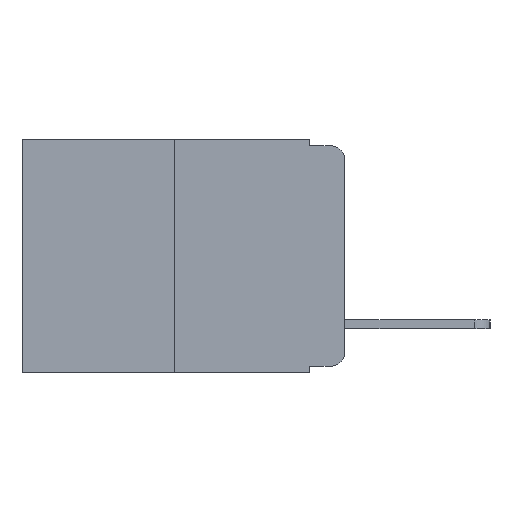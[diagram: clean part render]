
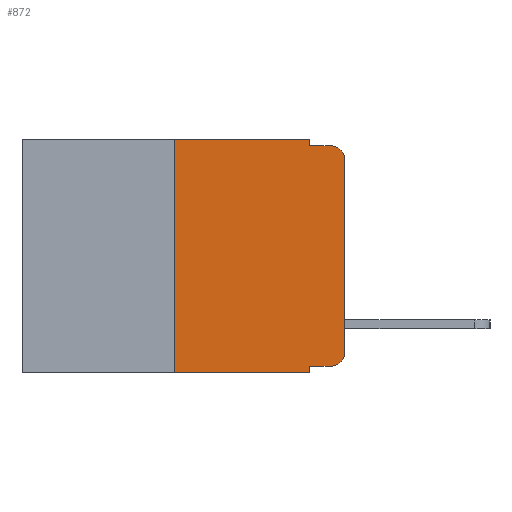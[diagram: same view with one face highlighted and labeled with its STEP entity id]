
A CAD part, left-side view. The second image highlights one B-rep face of the part: STEP entity #872.
In plain terms, the highlighted planar face has unit normal (-1, 0, 0).
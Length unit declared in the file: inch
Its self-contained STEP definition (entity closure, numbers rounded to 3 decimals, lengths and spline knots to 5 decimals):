
#131 = DIRECTION ( 'NONE',  ( 0., 0., -1. ) ) ;
#144 = EDGE_CURVE ( 'NONE', #8799, #7692, #14751, .T. ) ;
#221 = EDGE_LOOP ( 'NONE', ( #7815, #8333, #8622, #9562, #9704, #9836, #9785, #9309, #9465, #8725 ) ) ;
#251 = EDGE_CURVE ( 'NONE', #6473, #8799, #6221, .T. ) ;
#286 = CARTESIAN_POINT ( 'NONE',  ( 0., 0.051, 0. ) ) ;
#451 = VECTOR ( 'NONE', #1608, 39.37008 ) ;
#872 = ADVANCED_FACE ( 'NONE', ( #10704 ), #4887, .F. ) ;
#1161 = EDGE_CURVE ( 'NONE', #7692, #6128, #2024, .T. ) ;
#1162 = CARTESIAN_POINT ( 'NONE',  ( 0., 0.051, -0.343 ) ) ;
#1356 = CARTESIAN_POINT ( 'NONE',  ( 0., 0.25, 0. ) ) ;
#1543 = VERTEX_POINT ( 'NONE', #7859 ) ;
#1608 = DIRECTION ( 'NONE',  ( 0., 0., -1. ) ) ;
#1846 = CARTESIAN_POINT ( 'NONE',  ( 0., 0.02, -0.313 ) ) ;
#1879 = DIRECTION ( 'NONE',  ( 0., 0., 1. ) ) ;
#1979 = EDGE_CURVE ( 'NONE', #6128, #7221, #2002, .T. ) ;
#2002 = LINE ( 'NONE', #9554, #7936 ) ;
#2024 = LINE ( 'NONE', #8355, #13889 ) ;
#2084 = CARTESIAN_POINT ( 'NONE',  ( 0., 0.051, -0.333 ) ) ;
#2280 = CARTESIAN_POINT ( 'NONE',  ( 0., 0.473, 0. ) ) ;
#2773 = EDGE_CURVE ( 'NONE', #11988, #7221, #12708, .T. ) ;
#3029 = DIRECTION ( 'NONE',  ( 0., 0., -1. ) ) ;
#3569 = EDGE_CURVE ( 'NONE', #5573, #11988, #11482, .T. ) ;
#3654 = AXIS2_PLACEMENT_3D ( 'NONE', #1846, #10107, #3029 ) ;
#4259 = CARTESIAN_POINT ( 'NONE',  ( 0., 0., -0.313 ) ) ;
#4367 = DIRECTION ( 'NONE',  ( 0., -1., 0. ) ) ;
#4872 = EDGE_CURVE ( 'NONE', #6473, #12690, #12657, .T. ) ;
#4887 = PLANE ( 'NONE',  #13599 ) ;
#5160 = VERTEX_POINT ( 'NONE', #2084 ) ;
#5573 = VERTEX_POINT ( 'NONE', #4259 ) ;
#5961 = CARTESIAN_POINT ( 'NONE',  ( 0., 0., -0.03 ) ) ;
#6128 = VERTEX_POINT ( 'NONE', #11013 ) ;
#6221 = LINE ( 'NONE', #1356, #8914 ) ;
#6473 = VERTEX_POINT ( 'NONE', #9425 ) ;
#6611 = VECTOR ( 'NONE', #8003, 39.37008 ) ;
#6870 = CARTESIAN_POINT ( 'NONE',  ( 0., 0.473, -0.343 ) ) ;
#7221 = VERTEX_POINT ( 'NONE', #7530 ) ;
#7399 = DIRECTION ( 'NONE',  ( -1., 0., 0. ) ) ;
#7530 = CARTESIAN_POINT ( 'NONE',  ( 0., 0.02, -0.01 ) ) ;
#7692 = VERTEX_POINT ( 'NONE', #12306 ) ;
#7787 = CARTESIAN_POINT ( 'NONE',  ( 0., 0., 0. ) ) ;
#7815 = ORIENTED_EDGE ( 'NONE', *, *, #3569, .T. ) ;
#7859 = CARTESIAN_POINT ( 'NONE',  ( 0., 0.02, -0.333 ) ) ;
#7889 = CARTESIAN_POINT ( 'NONE',  ( 0., 0.051, -0.333 ) ) ;
#7936 = VECTOR ( 'NONE', #14992, 39.37008 ) ;
#8003 = DIRECTION ( 'NONE',  ( 0., -1., 0. ) ) ;
#8333 = ORIENTED_EDGE ( 'NONE', *, *, #2773, .T. ) ;
#8336 = DIRECTION ( 'NONE',  ( 0., 0., -1. ) ) ;
#8355 = CARTESIAN_POINT ( 'NONE',  ( 0., 0.051, 0. ) ) ;
#8438 = VECTOR ( 'NONE', #1879, 39.37008 ) ;
#8584 = VECTOR ( 'NONE', #11878, 39.37008 ) ;
#8622 = ORIENTED_EDGE ( 'NONE', *, *, #1979, .F. ) ;
#8725 = ORIENTED_EDGE ( 'NONE', *, *, #13129, .T. ) ;
#8799 = VERTEX_POINT ( 'NONE', #9569 ) ;
#8852 = LINE ( 'NONE', #7889, #14062 ) ;
#8914 = VECTOR ( 'NONE', #10843, 39.37008 ) ;
#9309 = ORIENTED_EDGE ( 'NONE', *, *, #14503, .F. ) ;
#9425 = CARTESIAN_POINT ( 'NONE',  ( 0., 0.25, -0.343 ) ) ;
#9465 = ORIENTED_EDGE ( 'NONE', *, *, #13816, .T. ) ;
#9554 = CARTESIAN_POINT ( 'NONE',  ( 0., 0.051, -0.01 ) ) ;
#9562 = ORIENTED_EDGE ( 'NONE', *, *, #1161, .F. ) ;
#9569 = CARTESIAN_POINT ( 'NONE',  ( 0., 0.25, 0. ) ) ;
#9704 = ORIENTED_EDGE ( 'NONE', *, *, #144, .F. ) ;
#9785 = ORIENTED_EDGE ( 'NONE', *, *, #4872, .T. ) ;
#9836 = ORIENTED_EDGE ( 'NONE', *, *, #251, .F. ) ;
#10107 = DIRECTION ( 'NONE',  ( -1., 0., 0. ) ) ;
#10704 = FACE_OUTER_BOUND ( 'NONE', #221, .T. ) ;
#10772 = CARTESIAN_POINT ( 'NONE',  ( 0., 0.473, 0. ) ) ;
#10843 = DIRECTION ( 'NONE',  ( 0., 0., 1. ) ) ;
#11013 = CARTESIAN_POINT ( 'NONE',  ( 0., 0.051, -0.01 ) ) ;
#11482 = LINE ( 'NONE', #7787, #8438 ) ;
#11878 = DIRECTION ( 'NONE',  ( 0., -1., 0. ) ) ;
#11988 = VERTEX_POINT ( 'NONE', #5961 ) ;
#12306 = CARTESIAN_POINT ( 'NONE',  ( 0., 0.051, 0. ) ) ;
#12364 = DIRECTION ( 'NONE',  ( 0., 0., -1. ) ) ;
#12657 = LINE ( 'NONE', #6870, #6611 ) ;
#12690 = VERTEX_POINT ( 'NONE', #1162 ) ;
#12708 = CIRCLE ( 'NONE', #14553, 0.02 ) ;
#12913 = LINE ( 'NONE', #286, #451 ) ;
#13037 = DIRECTION ( 'NONE',  ( 1., 0., 0. ) ) ;
#13129 = EDGE_CURVE ( 'NONE', #1543, #5573, #13420, .T. ) ;
#13420 = CIRCLE ( 'NONE', #3654, 0.02 ) ;
#13599 = AXIS2_PLACEMENT_3D ( 'NONE', #2280, #13037, #8336 ) ;
#13816 = EDGE_CURVE ( 'NONE', #5160, #1543, #8852, .T. ) ;
#13889 = VECTOR ( 'NONE', #12364, 39.37008 ) ;
#14062 = VECTOR ( 'NONE', #4367, 39.37008 ) ;
#14080 = CARTESIAN_POINT ( 'NONE',  ( 0., 0.02, -0.03 ) ) ;
#14503 = EDGE_CURVE ( 'NONE', #5160, #12690, #12913, .T. ) ;
#14553 = AXIS2_PLACEMENT_3D ( 'NONE', #14080, #7399, #131 ) ;
#14751 = LINE ( 'NONE', #10772, #8584 ) ;
#14992 = DIRECTION ( 'NONE',  ( 0., -1., 0. ) ) ;
